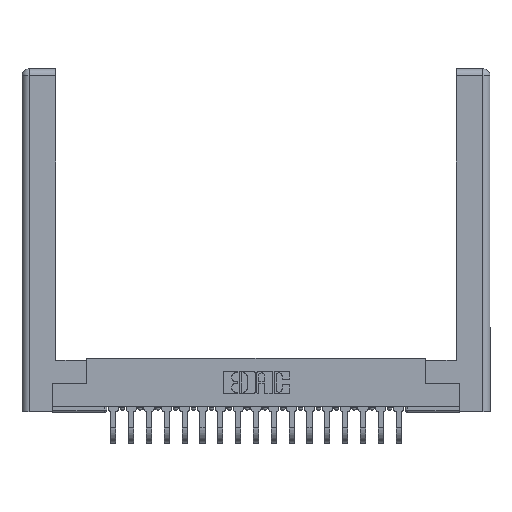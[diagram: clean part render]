
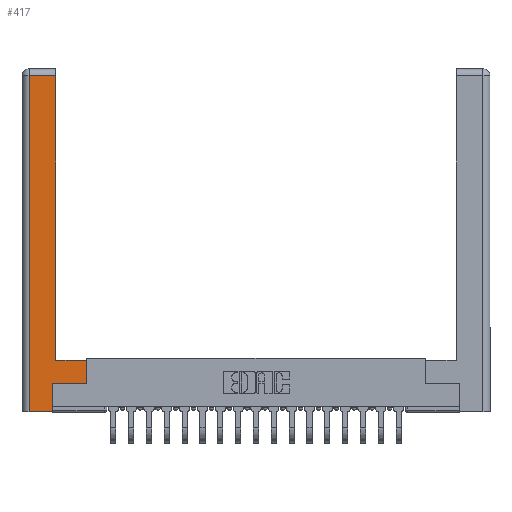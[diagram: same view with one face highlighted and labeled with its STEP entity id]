
A CAD part, top view. The second image highlights one B-rep face of the part: STEP entity #417.
In plain terms, the highlighted planar face has unit normal (0, 0, 1).
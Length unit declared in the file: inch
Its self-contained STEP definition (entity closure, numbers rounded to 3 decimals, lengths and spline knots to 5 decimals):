
#231 = ORIENTED_EDGE ( 'NONE', *, *, #9917, .T. ) ;
#417 = ADVANCED_FACE ( 'NONE', ( #17703 ), #13041, .F. ) ;
#636 = DIRECTION ( 'NONE',  ( -1., 0., 0. ) ) ;
#856 = VECTOR ( 'NONE', #2674, 39.37008 ) ;
#981 = CARTESIAN_POINT ( 'NONE',  ( 0.0615, 2.94, 0. ) ) ;
#1395 = ORIENTED_EDGE ( 'NONE', *, *, #19596, .T. ) ;
#2052 = CARTESIAN_POINT ( 'NONE',  ( 0.0615, 2.94, 0. ) ) ;
#2182 = VECTOR ( 'NONE', #8589, 39.37008 ) ;
#2200 = CARTESIAN_POINT ( 'NONE',  ( 0.295, 0.45, 0. ) ) ;
#2281 = LINE ( 'NONE', #10146, #7079 ) ;
#2674 = DIRECTION ( 'NONE',  ( 1., 0., 0. ) ) ;
#2785 = LINE ( 'NONE', #10539, #856 ) ;
#3246 = DIRECTION ( 'NONE',  ( 0., 0., -1. ) ) ;
#3312 = EDGE_CURVE ( 'NONE', #15984, #7698, #9851, .T. ) ;
#3820 = EDGE_CURVE ( 'NONE', #7698, #4196, #16628, .T. ) ;
#4133 = DIRECTION ( 'NONE',  ( 0., 1., 0. ) ) ;
#4196 = VERTEX_POINT ( 'NONE', #15040 ) ;
#4422 = VECTOR ( 'NONE', #20250, 39.37008 ) ;
#4950 = LINE ( 'NONE', #8069, #4422 ) ;
#5093 = VECTOR ( 'NONE', #17966, 39.37008 ) ;
#5898 = AXIS2_PLACEMENT_3D ( 'NONE', #9647, #3246, #19239 ) ;
#6485 = CARTESIAN_POINT ( 'NONE',  ( 0.565, 0.45, 0. ) ) ;
#6978 = VERTEX_POINT ( 'NONE', #8483 ) ;
#7079 = VECTOR ( 'NONE', #8586, 39.37008 ) ;
#7131 = DIRECTION ( 'NONE',  ( 0., 1., 0. ) ) ;
#7408 = CARTESIAN_POINT ( 'NONE',  ( 0.565, 0.245, 0. ) ) ;
#7698 = VERTEX_POINT ( 'NONE', #14118 ) ;
#8069 = CARTESIAN_POINT ( 'NONE',  ( 0.0615, 0., 0. ) ) ;
#8483 = CARTESIAN_POINT ( 'NONE',  ( 0.0615, 0., 0. ) ) ;
#8586 = DIRECTION ( 'NONE',  ( 1., 0., 0. ) ) ;
#8589 = DIRECTION ( 'NONE',  ( 0., 1., 0. ) ) ;
#8678 = VECTOR ( 'NONE', #636, 39.37008 ) ;
#8744 = CARTESIAN_POINT ( 'NONE',  ( 0.265, 0.245, 0. ) ) ;
#8954 = EDGE_LOOP ( 'NONE', ( #16321, #1395, #14932, #19746, #16247, #231, #10925, #17373 ) ) ;
#9647 = CARTESIAN_POINT ( 'NONE',  ( 0., 0., 0. ) ) ;
#9738 = VERTEX_POINT ( 'NONE', #16025 ) ;
#9851 = LINE ( 'NONE', #2200, #8678 ) ;
#9917 = EDGE_CURVE ( 'NONE', #18380, #12213, #2281, .T. ) ;
#10146 = CARTESIAN_POINT ( 'NONE',  ( 0.565, 0.245, 0. ) ) ;
#10539 = CARTESIAN_POINT ( 'NONE',  ( 0.265, 0., 0. ) ) ;
#10925 = ORIENTED_EDGE ( 'NONE', *, *, #12824, .T. ) ;
#11176 = EDGE_CURVE ( 'NONE', #9738, #18380, #19824, .T. ) ;
#11977 = VECTOR ( 'NONE', #7131, 39.37008 ) ;
#11998 = CARTESIAN_POINT ( 'NONE',  ( 0.265, 0.245, 0. ) ) ;
#12213 = VERTEX_POINT ( 'NONE', #7408 ) ;
#12824 = EDGE_CURVE ( 'NONE', #12213, #15984, #15062, .T. ) ;
#13041 = PLANE ( 'NONE',  #5898 ) ;
#14118 = CARTESIAN_POINT ( 'NONE',  ( 0.295, 0.45, 0. ) ) ;
#14177 = EDGE_CURVE ( 'NONE', #6978, #9738, #2785, .T. ) ;
#14932 = ORIENTED_EDGE ( 'NONE', *, *, #19569, .T. ) ;
#15040 = CARTESIAN_POINT ( 'NONE',  ( 0.295, 2.94, 0. ) ) ;
#15062 = LINE ( 'NONE', #19504, #18980 ) ;
#15984 = VERTEX_POINT ( 'NONE', #6485 ) ;
#16025 = CARTESIAN_POINT ( 'NONE',  ( 0.265, 0., 0. ) ) ;
#16191 = LINE ( 'NONE', #2052, #5093 ) ;
#16247 = ORIENTED_EDGE ( 'NONE', *, *, #11176, .T. ) ;
#16321 = ORIENTED_EDGE ( 'NONE', *, *, #3820, .T. ) ;
#16628 = LINE ( 'NONE', #19924, #11977 ) ;
#17373 = ORIENTED_EDGE ( 'NONE', *, *, #3312, .T. ) ;
#17703 = FACE_OUTER_BOUND ( 'NONE', #8954, .T. ) ;
#17966 = DIRECTION ( 'NONE',  ( -1., 0., 0. ) ) ;
#18380 = VERTEX_POINT ( 'NONE', #8744 ) ;
#18460 = VERTEX_POINT ( 'NONE', #981 ) ;
#18980 = VECTOR ( 'NONE', #4133, 39.37008 ) ;
#19239 = DIRECTION ( 'NONE',  ( -1., 0., 0. ) ) ;
#19504 = CARTESIAN_POINT ( 'NONE',  ( 0.565, 0.45, 0. ) ) ;
#19569 = EDGE_CURVE ( 'NONE', #18460, #6978, #4950, .T. ) ;
#19596 = EDGE_CURVE ( 'NONE', #4196, #18460, #16191, .T. ) ;
#19746 = ORIENTED_EDGE ( 'NONE', *, *, #14177, .T. ) ;
#19824 = LINE ( 'NONE', #11998, #2182 ) ;
#19924 = CARTESIAN_POINT ( 'NONE',  ( 0.295, 3., 0. ) ) ;
#20250 = DIRECTION ( 'NONE',  ( 0., -1., 0. ) ) ;
